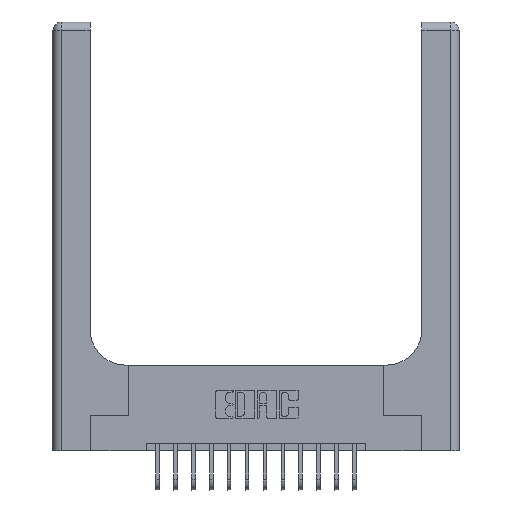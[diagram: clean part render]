
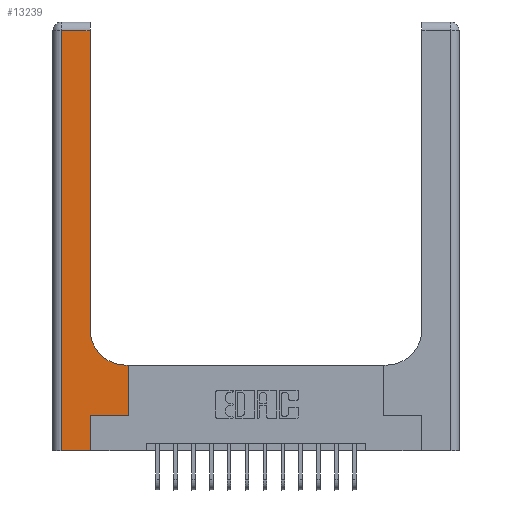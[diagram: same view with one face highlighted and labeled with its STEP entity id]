
A CAD part, top view. The second image highlights one B-rep face of the part: STEP entity #13239.
In plain terms, the highlighted planar face has unit normal (0, 0, 1).
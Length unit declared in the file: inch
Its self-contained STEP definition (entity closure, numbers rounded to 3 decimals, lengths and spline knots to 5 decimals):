
#9 = EDGE_CURVE ( 'NONE', #12352, #9155, #12290, .T. ) ;
#70 = VERTEX_POINT ( 'NONE', #8294 ) ;
#107 = CARTESIAN_POINT ( 'NONE',  ( 0.51, 0.85, 0.37 ) ) ;
#193 = ORIENTED_EDGE ( 'NONE', *, *, #14731, .T. ) ;
#612 = DIRECTION ( 'NONE',  ( 0., 1., 0. ) ) ;
#679 = VECTOR ( 'NONE', #4117, 39.37008 ) ;
#691 = CARTESIAN_POINT ( 'NONE',  ( 0., 2.94, 0.37 ) ) ;
#850 = DIRECTION ( 'NONE',  ( 0., 0., -1. ) ) ;
#856 = AXIS2_PLACEMENT_3D ( 'NONE', #12551, #850, #10076 ) ;
#893 = CARTESIAN_POINT ( 'NONE',  ( 0.06, 0., 0.37 ) ) ;
#1119 = VERTEX_POINT ( 'NONE', #8448 ) ;
#1474 = DIRECTION ( 'NONE',  ( 1., 0., 0. ) ) ;
#1661 = ORIENTED_EDGE ( 'NONE', *, *, #10509, .T. ) ;
#1730 = EDGE_CURVE ( 'NONE', #10424, #15294, #14390, .T. ) ;
#2065 = EDGE_CURVE ( 'NONE', #15294, #7554, #2651, .T. ) ;
#2279 = CARTESIAN_POINT ( 'NONE',  ( 0.06, 2.94, 0.37 ) ) ;
#2394 = EDGE_CURVE ( 'NONE', #3777, #70, #7835, .T. ) ;
#2651 = LINE ( 'NONE', #3927, #6628 ) ;
#3401 = DIRECTION ( 'NONE',  ( -1., 0., 0. ) ) ;
#3777 = VERTEX_POINT ( 'NONE', #9313 ) ;
#3787 = ORIENTED_EDGE ( 'NONE', *, *, #2394, .T. ) ;
#3927 = CARTESIAN_POINT ( 'NONE',  ( 0.265, 0., 0.37 ) ) ;
#4117 = DIRECTION ( 'NONE',  ( -1., 0., 0. ) ) ;
#5078 = CARTESIAN_POINT ( 'NONE',  ( 0.06, 3., 0.37 ) ) ;
#5481 = VECTOR ( 'NONE', #5625, 39.37008 ) ;
#5625 = DIRECTION ( 'NONE',  ( 0., 1., 0. ) ) ;
#5803 = CARTESIAN_POINT ( 'NONE',  ( 0.26, 2.94, 0.37 ) ) ;
#5948 = CARTESIAN_POINT ( 'NONE',  ( 0.528, 0.25, 0.37 ) ) ;
#5997 = CARTESIAN_POINT ( 'NONE',  ( 0.265, 0.25, 0.37 ) ) ;
#6114 = CARTESIAN_POINT ( 'NONE',  ( 0.265, 0., 0.37 ) ) ;
#6177 = PLANE ( 'NONE',  #856 ) ;
#6185 = EDGE_CURVE ( 'NONE', #1119, #12352, #14940, .T. ) ;
#6628 = VECTOR ( 'NONE', #11689, 39.37008 ) ;
#7554 = VERTEX_POINT ( 'NONE', #12066 ) ;
#7653 = VECTOR ( 'NONE', #14726, 39.37008 ) ;
#7769 = ORIENTED_EDGE ( 'NONE', *, *, #12390, .T. ) ;
#7835 = LINE ( 'NONE', #5948, #10826 ) ;
#8294 = CARTESIAN_POINT ( 'NONE',  ( 0.528, 0.6, 0.37 ) ) ;
#8448 = CARTESIAN_POINT ( 'NONE',  ( 0.51, 0.6, 0.37 ) ) ;
#8490 = EDGE_LOOP ( 'NONE', ( #13195, #193, #1661, #13436, #10457, #15671, #3787, #7769, #9683 ) ) ;
#8499 = VECTOR ( 'NONE', #3401, 39.37008 ) ;
#9155 = VERTEX_POINT ( 'NONE', #5803 ) ;
#9301 = VERTEX_POINT ( 'NONE', #2279 ) ;
#9313 = CARTESIAN_POINT ( 'NONE',  ( 0.528, 0.25, 0.37 ) ) ;
#9361 = FACE_OUTER_BOUND ( 'NONE', #8490, .T. ) ;
#9400 = DIRECTION ( 'NONE',  ( 0., 0., -1. ) ) ;
#9683 = ORIENTED_EDGE ( 'NONE', *, *, #6185, .T. ) ;
#10076 = DIRECTION ( 'NONE',  ( -1., 0., 0. ) ) ;
#10424 = VERTEX_POINT ( 'NONE', #893 ) ;
#10457 = ORIENTED_EDGE ( 'NONE', *, *, #2065, .T. ) ;
#10509 = EDGE_CURVE ( 'NONE', #9301, #10424, #10994, .T. ) ;
#10544 = CARTESIAN_POINT ( 'NONE',  ( 0.26, 0.85, 0.37 ) ) ;
#10826 = VECTOR ( 'NONE', #612, 39.37008 ) ;
#10982 = CARTESIAN_POINT ( 'NONE',  ( 0., 0., 0.37 ) ) ;
#10994 = LINE ( 'NONE', #5078, #13954 ) ;
#11354 = EDGE_CURVE ( 'NONE', #7554, #3777, #12776, .T. ) ;
#11689 = DIRECTION ( 'NONE',  ( 0., 1., 0. ) ) ;
#12066 = CARTESIAN_POINT ( 'NONE',  ( 0.265, 0.25, 0.37 ) ) ;
#12290 = LINE ( 'NONE', #16643, #5481 ) ;
#12352 = VERTEX_POINT ( 'NONE', #10544 ) ;
#12390 = EDGE_CURVE ( 'NONE', #70, #1119, #13709, .T. ) ;
#12551 = CARTESIAN_POINT ( 'NONE',  ( 0., 3., 0.37 ) ) ;
#12667 = LINE ( 'NONE', #691, #8499 ) ;
#12776 = LINE ( 'NONE', #5997, #13184 ) ;
#13151 = CARTESIAN_POINT ( 'NONE',  ( 0.26, 0.6, 0.37 ) ) ;
#13184 = VECTOR ( 'NONE', #13651, 39.37008 ) ;
#13195 = ORIENTED_EDGE ( 'NONE', *, *, #9, .T. ) ;
#13239 = ADVANCED_FACE ( 'NONE', ( #9361 ), #6177, .F. ) ;
#13436 = ORIENTED_EDGE ( 'NONE', *, *, #1730, .T. ) ;
#13651 = DIRECTION ( 'NONE',  ( 1., 0., 0. ) ) ;
#13709 = LINE ( 'NONE', #13151, #679 ) ;
#13853 = AXIS2_PLACEMENT_3D ( 'NONE', #107, #9400, #1474 ) ;
#13954 = VECTOR ( 'NONE', #15291, 39.37008 ) ;
#14390 = LINE ( 'NONE', #10982, #7653 ) ;
#14726 = DIRECTION ( 'NONE',  ( 1., 0., 0. ) ) ;
#14731 = EDGE_CURVE ( 'NONE', #9155, #9301, #12667, .T. ) ;
#14940 = CIRCLE ( 'NONE', #13853, 0.25 ) ;
#15291 = DIRECTION ( 'NONE',  ( 0., -1., 0. ) ) ;
#15294 = VERTEX_POINT ( 'NONE', #6114 ) ;
#15671 = ORIENTED_EDGE ( 'NONE', *, *, #11354, .T. ) ;
#16643 = CARTESIAN_POINT ( 'NONE',  ( 0.26, 3., 0.37 ) ) ;
